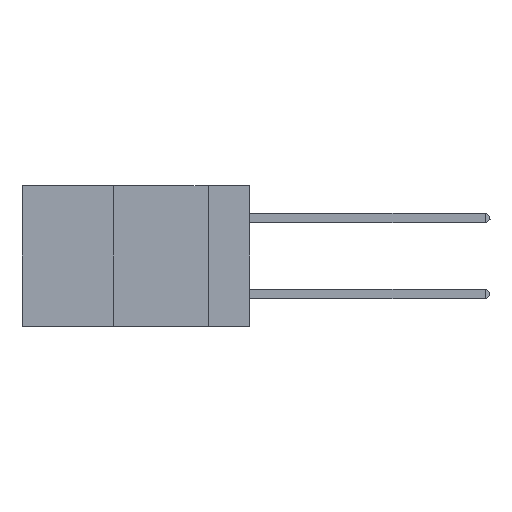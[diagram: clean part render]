
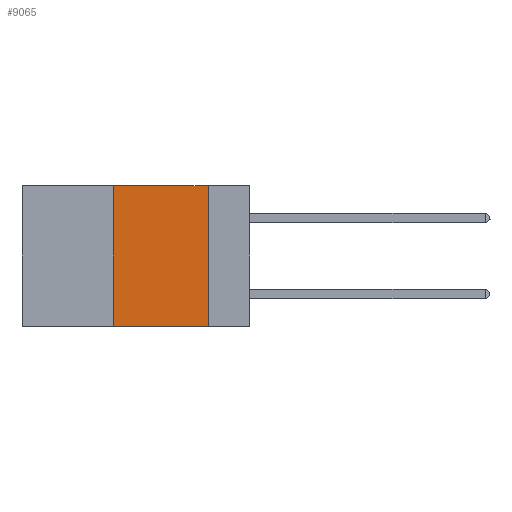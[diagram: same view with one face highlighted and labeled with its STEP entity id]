
A CAD part, left-side view. The second image highlights one B-rep face of the part: STEP entity #9065.
In plain terms, the highlighted planar face has unit normal (-1, 0, 0).
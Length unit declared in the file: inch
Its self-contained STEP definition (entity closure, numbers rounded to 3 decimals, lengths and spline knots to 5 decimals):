
#837 = ORIENTED_EDGE ( 'NONE', *, *, #12439, .T. ) ;
#1795 = CARTESIAN_POINT ( 'NONE',  ( 0., 0.36, 0. ) ) ;
#1863 = ORIENTED_EDGE ( 'NONE', *, *, #5693, .F. ) ;
#2936 = CARTESIAN_POINT ( 'NONE',  ( 0., 0.6, 0. ) ) ;
#3375 = VERTEX_POINT ( 'NONE', #11145 ) ;
#3395 = ORIENTED_EDGE ( 'NONE', *, *, #6277, .F. ) ;
#3644 = VECTOR ( 'NONE', #13411, 39.37008 ) ;
#3669 = LINE ( 'NONE', #11203, #3644 ) ;
#3894 = EDGE_LOOP ( 'NONE', ( #3395, #6225, #1863, #837 ) ) ;
#4468 = DIRECTION ( 'NONE',  ( 0., -1., 0. ) ) ;
#4764 = VECTOR ( 'NONE', #9347, 39.37008 ) ;
#5205 = EDGE_CURVE ( 'NONE', #7432, #8889, #10418, .T. ) ;
#5693 = EDGE_CURVE ( 'NONE', #9797, #7432, #9329, .T. ) ;
#6225 = ORIENTED_EDGE ( 'NONE', *, *, #5205, .F. ) ;
#6277 = EDGE_CURVE ( 'NONE', #8889, #3375, #3669, .T. ) ;
#7432 = VERTEX_POINT ( 'NONE', #9775 ) ;
#7818 = AXIS2_PLACEMENT_3D ( 'NONE', #11554, #13950, #11823 ) ;
#8889 = VERTEX_POINT ( 'NONE', #11271 ) ;
#8891 = CARTESIAN_POINT ( 'NONE',  ( 0., 0.36, -0.37 ) ) ;
#8950 = LINE ( 'NONE', #12373, #13796 ) ;
#9065 = ADVANCED_FACE ( 'NONE', ( #12886 ), #9416, .F. ) ;
#9329 = LINE ( 'NONE', #1795, #9774 ) ;
#9347 = DIRECTION ( 'NONE',  ( 0., -1., 0. ) ) ;
#9416 = PLANE ( 'NONE',  #7818 ) ;
#9774 = VECTOR ( 'NONE', #11602, 39.37008 ) ;
#9775 = CARTESIAN_POINT ( 'NONE',  ( 0., 0.36, 0. ) ) ;
#9797 = VERTEX_POINT ( 'NONE', #8891 ) ;
#10418 = LINE ( 'NONE', #2936, #4764 ) ;
#11145 = CARTESIAN_POINT ( 'NONE',  ( 0., 0.11, -0.37 ) ) ;
#11203 = CARTESIAN_POINT ( 'NONE',  ( 0., 0.11, 0. ) ) ;
#11271 = CARTESIAN_POINT ( 'NONE',  ( 0., 0.11, 0. ) ) ;
#11554 = CARTESIAN_POINT ( 'NONE',  ( 0., 0.6, 0. ) ) ;
#11602 = DIRECTION ( 'NONE',  ( 0., 0., 1. ) ) ;
#11823 = DIRECTION ( 'NONE',  ( 0., 0., -1. ) ) ;
#12373 = CARTESIAN_POINT ( 'NONE',  ( 0., 0.6, -0.37 ) ) ;
#12439 = EDGE_CURVE ( 'NONE', #9797, #3375, #8950, .T. ) ;
#12886 = FACE_OUTER_BOUND ( 'NONE', #3894, .T. ) ;
#13411 = DIRECTION ( 'NONE',  ( 0., 0., -1. ) ) ;
#13796 = VECTOR ( 'NONE', #4468, 39.37008 ) ;
#13950 = DIRECTION ( 'NONE',  ( 1., 0., 0. ) ) ;
